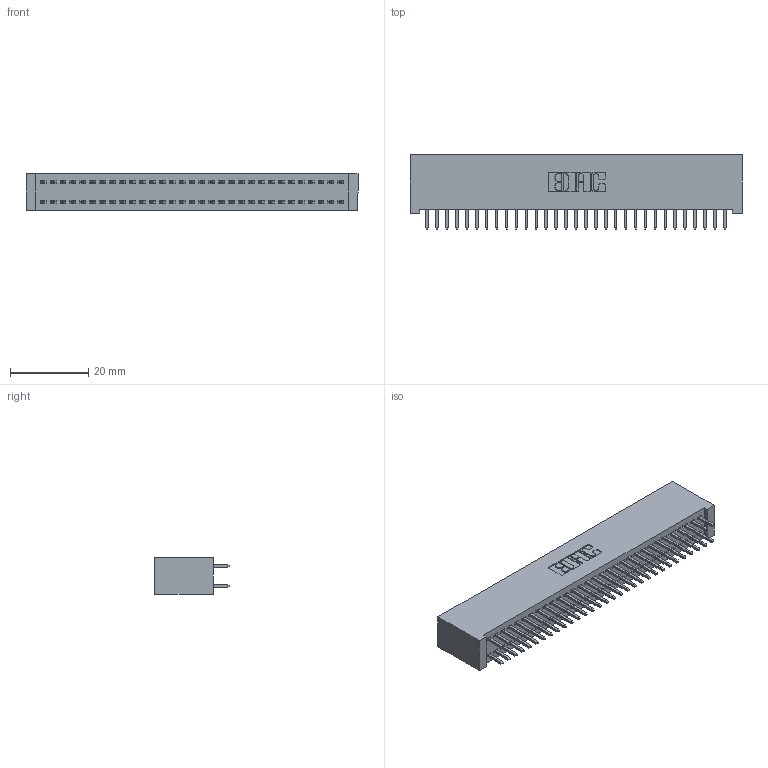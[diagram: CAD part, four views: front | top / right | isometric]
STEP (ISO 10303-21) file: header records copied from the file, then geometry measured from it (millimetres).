
FILE_DESCRIPTION (( 'STEP AP203' ), '1' );
FILE_NAME ('342-062-521-201.STEP', '2019-10-03T13:44:58', ( '' ), ( '' ), 'SwSTEP 2.0', 'SolidWorks 2016', '' );
FILE_SCHEMA (( 'CONFIG_CONTROL_DESIGN' ));
Length unit declared in the file: inch
Products named in the file (3): 342 Part_Lugless; 345-292-001_345-293-121; 342-062-521-201
Assembly tree (63 placements, depth 2):
  342-062-521-201
    342 Part_Lugless
    345-292-001_345-293-121  x62
Bounding box: 84.99 x 19.06 x 9.4 mm (x, y, z)
Volume: 7998.3 mm3; surface area: 13023.1 mm2
Topology: 63 solids, 63 shells, 3326 faces, 9885 edges, 6506 vertices
Faces by surface type: plane 2294, cylinder 1032
Entity records: 20975 total; most frequent: CARTESIAN_POINT 3486, ORIENTED_EDGE 3422, DIRECTION 2991, EDGE_CURVE 1711, VECTOR 1591, LINE 1591, VERTEX_POINT 1138, AXIS2_PLACEMENT_3D 700
